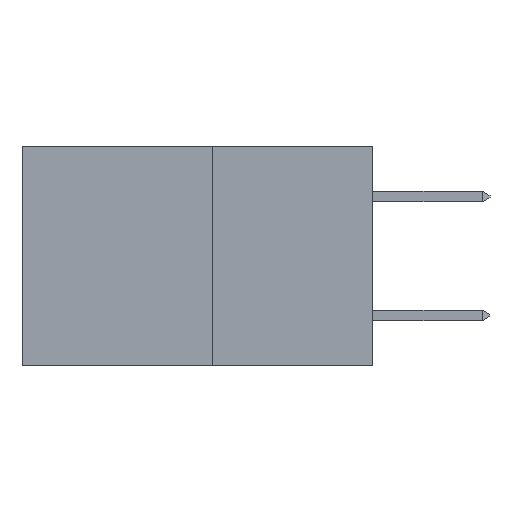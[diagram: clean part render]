
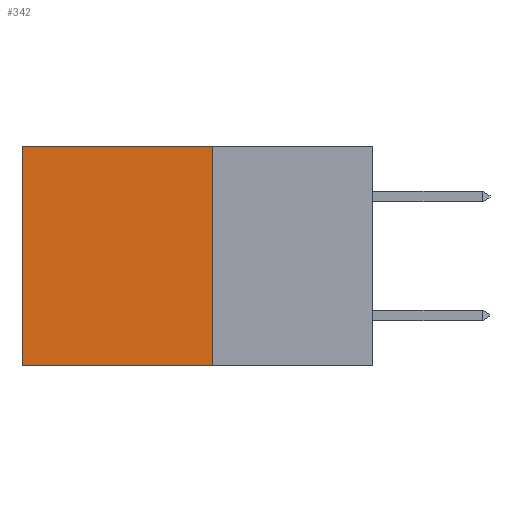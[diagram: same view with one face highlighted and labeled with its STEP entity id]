
A CAD part, left-side view. The second image highlights one B-rep face of the part: STEP entity #342.
In plain terms, the highlighted planar face has unit normal (-1, 0, 0).
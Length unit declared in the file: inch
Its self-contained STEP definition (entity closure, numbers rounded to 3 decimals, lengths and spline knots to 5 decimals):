
#59 = CARTESIAN_POINT ( 'NONE',  ( 0.277, 0.59, -0.37 ) ) ;
#162 = VERTEX_POINT ( 'NONE', #4929 ) ;
#237 = EDGE_CURVE ( 'NONE', #1579, #162, #6530, .T. ) ;
#257 = ORIENTED_EDGE ( 'NONE', *, *, #5050, .F. ) ;
#342 = ADVANCED_FACE ( 'NONE', ( #5804 ), #6751, .F. ) ;
#558 = VECTOR ( 'NONE', #1981, 39.37008 ) ;
#730 = VECTOR ( 'NONE', #3425, 39.37008 ) ;
#935 = LINE ( 'NONE', #7269, #7325 ) ;
#1415 = EDGE_CURVE ( 'NONE', #7915, #162, #7035, .T. ) ;
#1579 = VERTEX_POINT ( 'NONE', #6881 ) ;
#1981 = DIRECTION ( 'NONE',  ( 0., 0., -1. ) ) ;
#2194 = VERTEX_POINT ( 'NONE', #3636 ) ;
#2775 = ORIENTED_EDGE ( 'NONE', *, *, #1415, .T. ) ;
#3012 = DIRECTION ( 'NONE',  ( 0., 1., 0. ) ) ;
#3425 = DIRECTION ( 'NONE',  ( 0., 0., -1. ) ) ;
#3636 = CARTESIAN_POINT ( 'NONE',  ( 0.277, 0.27, 0. ) ) ;
#4617 = CARTESIAN_POINT ( 'NONE',  ( 0.277, 0.27, -0.37 ) ) ;
#4699 = CARTESIAN_POINT ( 'NONE',  ( 0.277, 0.59, 0. ) ) ;
#4929 = CARTESIAN_POINT ( 'NONE',  ( 0.277, 0.59, -0.37 ) ) ;
#5044 = ORIENTED_EDGE ( 'NONE', *, *, #6786, .T. ) ;
#5050 = EDGE_CURVE ( 'NONE', #2194, #1579, #7343, .T. ) ;
#5804 = FACE_OUTER_BOUND ( 'NONE', #7077, .T. ) ;
#5976 = DIRECTION ( 'NONE',  ( 1., 0., 0. ) ) ;
#6158 = DIRECTION ( 'NONE',  ( 0., 0., -1. ) ) ;
#6224 = ORIENTED_EDGE ( 'NONE', *, *, #237, .F. ) ;
#6530 = LINE ( 'NONE', #4617, #6695 ) ;
#6638 = AXIS2_PLACEMENT_3D ( 'NONE', #6727, #5976, #6158 ) ;
#6695 = VECTOR ( 'NONE', #7692, 39.37008 ) ;
#6727 = CARTESIAN_POINT ( 'NONE',  ( 0.277, 0.27, -0.37 ) ) ;
#6751 = PLANE ( 'NONE',  #6638 ) ;
#6786 = EDGE_CURVE ( 'NONE', #2194, #7915, #935, .T. ) ;
#6881 = CARTESIAN_POINT ( 'NONE',  ( 0.277, 0.27, -0.37 ) ) ;
#7035 = LINE ( 'NONE', #59, #558 ) ;
#7077 = EDGE_LOOP ( 'NONE', ( #2775, #6224, #257, #5044 ) ) ;
#7269 = CARTESIAN_POINT ( 'NONE',  ( 0.277, 0.27, 0. ) ) ;
#7325 = VECTOR ( 'NONE', #3012, 39.37008 ) ;
#7343 = LINE ( 'NONE', #8007, #730 ) ;
#7692 = DIRECTION ( 'NONE',  ( 0., 1., 0. ) ) ;
#7915 = VERTEX_POINT ( 'NONE', #4699 ) ;
#8007 = CARTESIAN_POINT ( 'NONE',  ( 0.277, 0.27, -0.37 ) ) ;
